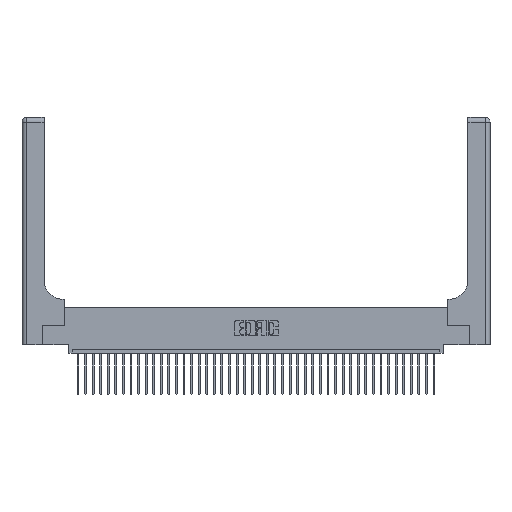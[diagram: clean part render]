
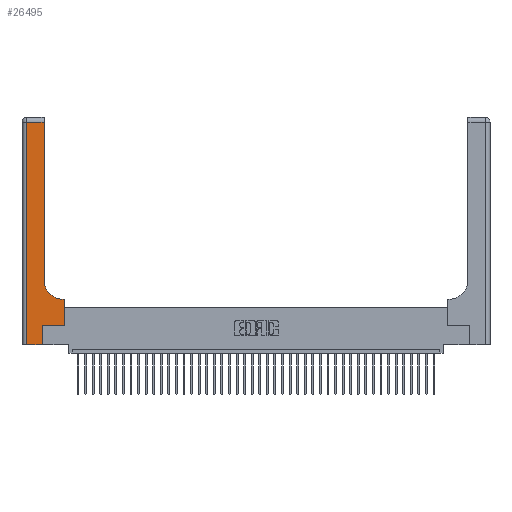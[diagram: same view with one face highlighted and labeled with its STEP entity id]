
A CAD part, top view. The second image highlights one B-rep face of the part: STEP entity #26495.
In plain terms, the highlighted planar face has unit normal (0, 0, 1).
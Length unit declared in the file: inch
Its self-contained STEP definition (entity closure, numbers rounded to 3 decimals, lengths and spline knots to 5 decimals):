
#183 = DIRECTION ( 'NONE',  ( 0., 1., 0. ) ) ;
#202 = DIRECTION ( 'NONE',  ( -1., 0., 0. ) ) ;
#1065 = VERTEX_POINT ( 'NONE', #17492 ) ;
#1253 = DIRECTION ( 'NONE',  ( 0., 1., 0. ) ) ;
#1318 = CARTESIAN_POINT ( 'NONE',  ( 0.269, 0., 0.37 ) ) ;
#2550 = VERTEX_POINT ( 'NONE', #6504 ) ;
#3123 = CARTESIAN_POINT ( 'NONE',  ( 0.2915, 0.85, 0.37 ) ) ;
#3331 = CARTESIAN_POINT ( 'NONE',  ( 0.5585, 0.25, 0.37 ) ) ;
#3868 = CARTESIAN_POINT ( 'NONE',  ( 0.2915, 3., 0.37 ) ) ;
#4439 = VECTOR ( 'NONE', #7786, 39.37008 ) ;
#5043 = VERTEX_POINT ( 'NONE', #31078 ) ;
#5635 = DIRECTION ( 'NONE',  ( -1., 0., 0. ) ) ;
#6019 = ORIENTED_EDGE ( 'NONE', *, *, #34318, .T. ) ;
#6504 = CARTESIAN_POINT ( 'NONE',  ( 0.5585, 0.25, 0.37 ) ) ;
#7786 = DIRECTION ( 'NONE',  ( 1., 0., 0. ) ) ;
#8527 = PLANE ( 'NONE',  #24611 ) ;
#8668 = LINE ( 'NONE', #38312, #29666 ) ;
#8821 = LINE ( 'NONE', #3868, #10800 ) ;
#8998 = DIRECTION ( 'NONE',  ( 0., 0., -1. ) ) ;
#9212 = CARTESIAN_POINT ( 'NONE',  ( 0.269, 0.25, 0.37 ) ) ;
#10800 = VECTOR ( 'NONE', #1253, 39.37008 ) ;
#11138 = ORIENTED_EDGE ( 'NONE', *, *, #33842, .T. ) ;
#11980 = CARTESIAN_POINT ( 'NONE',  ( 0., 3., 0.37 ) ) ;
#12016 = EDGE_CURVE ( 'NONE', #14209, #2550, #22087, .T. ) ;
#14209 = VERTEX_POINT ( 'NONE', #9212 ) ;
#14568 = CARTESIAN_POINT ( 'NONE',  ( 0.06, 3., 0.37 ) ) ;
#15709 = CARTESIAN_POINT ( 'NONE',  ( 0.5415, 0.85, 0.37 ) ) ;
#15896 = CARTESIAN_POINT ( 'NONE',  ( 0., 0., 0.37 ) ) ;
#17492 = CARTESIAN_POINT ( 'NONE',  ( 0.2915, 2.94, 0.37 ) ) ;
#17691 = DIRECTION ( 'NONE',  ( 0., -1., 0. ) ) ;
#18617 = LINE ( 'NONE', #21381, #24030 ) ;
#19316 = DIRECTION ( 'NONE',  ( 1., 0., 0. ) ) ;
#20077 = VERTEX_POINT ( 'NONE', #1318 ) ;
#20485 = ORIENTED_EDGE ( 'NONE', *, *, #12016, .T. ) ;
#21381 = CARTESIAN_POINT ( 'NONE',  ( 0.269, 0., 0.37 ) ) ;
#21579 = ORIENTED_EDGE ( 'NONE', *, *, #26328, .T. ) ;
#21832 = EDGE_CURVE ( 'NONE', #2550, #24075, #22232, .T. ) ;
#22087 = LINE ( 'NONE', #32447, #4439 ) ;
#22232 = LINE ( 'NONE', #3331, #39911 ) ;
#22455 = ORIENTED_EDGE ( 'NONE', *, *, #25692, .T. ) ;
#22598 = LINE ( 'NONE', #24719, #38302 ) ;
#23850 = VERTEX_POINT ( 'NONE', #34866 ) ;
#24030 = VECTOR ( 'NONE', #30289, 39.37008 ) ;
#24075 = VERTEX_POINT ( 'NONE', #40326 ) ;
#24611 = AXIS2_PLACEMENT_3D ( 'NONE', #11980, #30757, #5635 ) ;
#24719 = CARTESIAN_POINT ( 'NONE',  ( 0., 2.94, 0.37 ) ) ;
#25017 = ORIENTED_EDGE ( 'NONE', *, *, #25983, .T. ) ;
#25692 = EDGE_CURVE ( 'NONE', #1065, #23850, #22598, .T. ) ;
#25983 = EDGE_CURVE ( 'NONE', #27031, #20077, #28493, .T. ) ;
#26328 = EDGE_CURVE ( 'NONE', #39055, #1065, #8821, .T. ) ;
#26495 = ADVANCED_FACE ( 'NONE', ( #33376 ), #8527, .F. ) ;
#27031 = VERTEX_POINT ( 'NONE', #30201 ) ;
#27895 = AXIS2_PLACEMENT_3D ( 'NONE', #15709, #8998, #37630 ) ;
#28493 = LINE ( 'NONE', #15896, #30473 ) ;
#29666 = VECTOR ( 'NONE', #202, 39.37008 ) ;
#30201 = CARTESIAN_POINT ( 'NONE',  ( 0.06, 0., 0.37 ) ) ;
#30289 = DIRECTION ( 'NONE',  ( 0., 1., 0. ) ) ;
#30449 = ORIENTED_EDGE ( 'NONE', *, *, #31075, .T. ) ;
#30473 = VECTOR ( 'NONE', #19316, 39.37008 ) ;
#30595 = EDGE_LOOP ( 'NONE', ( #21579, #22455, #6019, #25017, #37543, #20485, #37003, #30449, #11138 ) ) ;
#30757 = DIRECTION ( 'NONE',  ( 0., 0., -1. ) ) ;
#31075 = EDGE_CURVE ( 'NONE', #24075, #5043, #8668, .T. ) ;
#31078 = CARTESIAN_POINT ( 'NONE',  ( 0.5415, 0.6, 0.37 ) ) ;
#31826 = CIRCLE ( 'NONE', #27895, 0.25 ) ;
#32308 = VECTOR ( 'NONE', #17691, 39.37008 ) ;
#32447 = CARTESIAN_POINT ( 'NONE',  ( 0.269, 0.25, 0.37 ) ) ;
#33376 = FACE_OUTER_BOUND ( 'NONE', #30595, .T. ) ;
#33842 = EDGE_CURVE ( 'NONE', #5043, #39055, #31826, .T. ) ;
#34318 = EDGE_CURVE ( 'NONE', #23850, #27031, #37708, .T. ) ;
#34328 = EDGE_CURVE ( 'NONE', #20077, #14209, #18617, .T. ) ;
#34866 = CARTESIAN_POINT ( 'NONE',  ( 0.06, 2.94, 0.37 ) ) ;
#37003 = ORIENTED_EDGE ( 'NONE', *, *, #21832, .T. ) ;
#37543 = ORIENTED_EDGE ( 'NONE', *, *, #34328, .T. ) ;
#37630 = DIRECTION ( 'NONE',  ( 1., 0., 0. ) ) ;
#37708 = LINE ( 'NONE', #14568, #32308 ) ;
#38302 = VECTOR ( 'NONE', #40089, 39.37008 ) ;
#38312 = CARTESIAN_POINT ( 'NONE',  ( 0.2915, 0.6, 0.37 ) ) ;
#39055 = VERTEX_POINT ( 'NONE', #3123 ) ;
#39911 = VECTOR ( 'NONE', #183, 39.37008 ) ;
#40089 = DIRECTION ( 'NONE',  ( -1., 0., 0. ) ) ;
#40326 = CARTESIAN_POINT ( 'NONE',  ( 0.5585, 0.6, 0.37 ) ) ;
